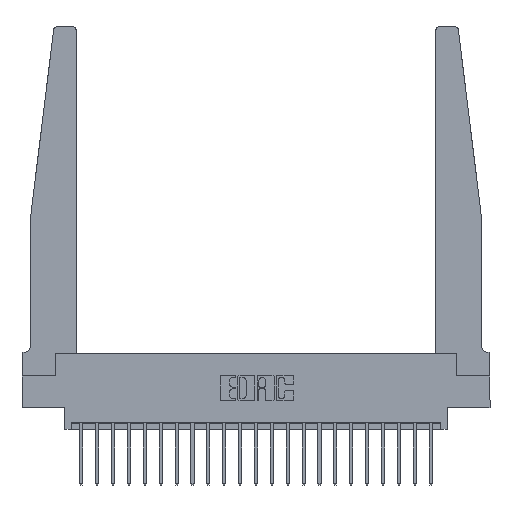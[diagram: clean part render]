
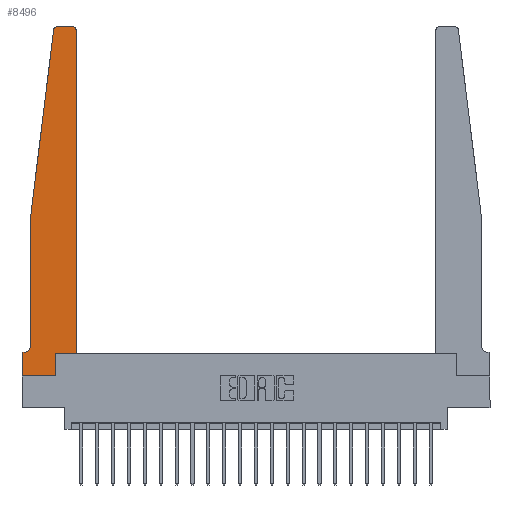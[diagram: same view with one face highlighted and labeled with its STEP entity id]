
A CAD part, top view. The second image highlights one B-rep face of the part: STEP entity #8496.
In plain terms, the highlighted planar face has unit normal (0, 0, 1).
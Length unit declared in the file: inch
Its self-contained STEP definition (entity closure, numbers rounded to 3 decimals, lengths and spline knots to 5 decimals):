
#109 = EDGE_LOOP ( 'NONE', ( #13309, #15903, #14687, #2676, #15433, #5924, #4441, #11190, #1100, #531, #7987, #18024 ) ) ;
#251 = CARTESIAN_POINT ( 'NONE',  ( 0.425, 2.72, 0.37 ) ) ;
#488 = EDGE_CURVE ( 'NONE', #21407, #11860, #6387, .T. ) ;
#531 = ORIENTED_EDGE ( 'NONE', *, *, #16095, .T. ) ;
#1100 = ORIENTED_EDGE ( 'NONE', *, *, #2071, .T. ) ;
#1264 = DIRECTION ( 'NONE',  ( -1., 0., 0. ) ) ;
#1304 = VECTOR ( 'NONE', #15452, 39.37008 ) ;
#2071 = EDGE_CURVE ( 'NONE', #9517, #12862, #4675, .T. ) ;
#2253 = CARTESIAN_POINT ( 'NONE',  ( 0., 0., 0.37 ) ) ;
#2350 = CIRCLE ( 'NONE', #16091, 0.05 ) ;
#2676 = ORIENTED_EDGE ( 'NONE', *, *, #9889, .T. ) ;
#2680 = VERTEX_POINT ( 'NONE', #2723 ) ;
#2683 = DIRECTION ( 'NONE',  ( 1., 0., 0. ) ) ;
#2723 = CARTESIAN_POINT ( 'NONE',  ( 0., 0.1875, 0.37 ) ) ;
#3309 = DIRECTION ( 'NONE',  ( 0., 0., 1. ) ) ;
#3748 = EDGE_CURVE ( 'NONE', #21565, #18708, #15026, .T. ) ;
#3820 = LINE ( 'NONE', #15959, #9066 ) ;
#4441 = ORIENTED_EDGE ( 'NONE', *, *, #20902, .T. ) ;
#4668 = CARTESIAN_POINT ( 'NONE',  ( 0.395, 2.72, 0.37 ) ) ;
#4675 = LINE ( 'NONE', #7971, #13459 ) ;
#4796 = CARTESIAN_POINT ( 'NONE',  ( 0.065, 1.25, 0.37 ) ) ;
#5577 = CARTESIAN_POINT ( 'NONE',  ( 0., 0., 0.37 ) ) ;
#5736 = CARTESIAN_POINT ( 'NONE',  ( 0.2605, 0.18, 0.37 ) ) ;
#5771 = CARTESIAN_POINT ( 'NONE',  ( 0.2605, 0., 0.37 ) ) ;
#5870 = LINE ( 'NONE', #11417, #14626 ) ;
#5924 = ORIENTED_EDGE ( 'NONE', *, *, #21323, .T. ) ;
#6345 = CARTESIAN_POINT ( 'NONE',  ( 0., 0., 0.37 ) ) ;
#6387 = LINE ( 'NONE', #19167, #15132 ) ;
#6426 = DIRECTION ( 'NONE',  ( 1., 0., 0. ) ) ;
#6917 = EDGE_CURVE ( 'NONE', #17270, #9517, #17255, .T. ) ;
#6974 = EDGE_CURVE ( 'NONE', #11742, #21407, #16705, .T. ) ;
#7062 = LINE ( 'NONE', #20667, #20421 ) ;
#7329 = DIRECTION ( 'NONE',  ( 0., -1., 0. ) ) ;
#7659 = LINE ( 'NONE', #5577, #16386 ) ;
#7971 = CARTESIAN_POINT ( 'NONE',  ( 0.2605, 0.18, 0.37 ) ) ;
#7987 = ORIENTED_EDGE ( 'NONE', *, *, #19603, .T. ) ;
#8454 = CARTESIAN_POINT ( 'NONE',  ( 0.25, 2.75, 0.37 ) ) ;
#8496 = ADVANCED_FACE ( 'NONE', ( #18513 ), #13808, .T. ) ;
#8518 = CARTESIAN_POINT ( 'NONE',  ( 0., 0.1875, 0.37 ) ) ;
#9066 = VECTOR ( 'NONE', #21141, 39.37008 ) ;
#9517 = VERTEX_POINT ( 'NONE', #5771 ) ;
#9761 = DIRECTION ( 'NONE',  ( 0., 1., 0. ) ) ;
#9889 = EDGE_CURVE ( 'NONE', #11860, #9933, #7062, .T. ) ;
#9890 = DIRECTION ( 'NONE',  ( 1., 0., 0. ) ) ;
#9933 = VERTEX_POINT ( 'NONE', #20735 ) ;
#10051 = CARTESIAN_POINT ( 'NONE',  ( 0.27653, 2.72, 0.37 ) ) ;
#10329 = DIRECTION ( 'NONE',  ( 0., -1., 0. ) ) ;
#11150 = VERTEX_POINT ( 'NONE', #20262 ) ;
#11190 = ORIENTED_EDGE ( 'NONE', *, *, #6917, .T. ) ;
#11417 = CARTESIAN_POINT ( 'NONE',  ( 0.425, 0.18, 0.37 ) ) ;
#11742 = VERTEX_POINT ( 'NONE', #13229 ) ;
#11788 = DIRECTION ( 'NONE',  ( 0., 0., -1. ) ) ;
#11811 = DIRECTION ( 'NONE',  ( 1., 0., 0. ) ) ;
#11853 = EDGE_CURVE ( 'NONE', #9933, #12474, #2350, .T. ) ;
#11860 = VERTEX_POINT ( 'NONE', #4796 ) ;
#11968 = CARTESIAN_POINT ( 'NONE',  ( 0.065, 0.1875, 0.37 ) ) ;
#12474 = VERTEX_POINT ( 'NONE', #22196 ) ;
#12680 = VECTOR ( 'NONE', #9890, 39.37008 ) ;
#12862 = VERTEX_POINT ( 'NONE', #5736 ) ;
#12879 = LINE ( 'NONE', #11968, #21466 ) ;
#13229 = CARTESIAN_POINT ( 'NONE',  ( 0.27653, 2.75, 0.37 ) ) ;
#13309 = ORIENTED_EDGE ( 'NONE', *, *, #22333, .T. ) ;
#13459 = VECTOR ( 'NONE', #9761, 39.37008 ) ;
#13808 = PLANE ( 'NONE',  #15047 ) ;
#13932 = CARTESIAN_POINT ( 'NONE',  ( 0.24675, 2.72367, 0.37 ) ) ;
#14626 = VECTOR ( 'NONE', #2683, 39.37008 ) ;
#14687 = ORIENTED_EDGE ( 'NONE', *, *, #488, .T. ) ;
#14810 = CARTESIAN_POINT ( 'NONE',  ( 0.395, 2.75, 0.37 ) ) ;
#15026 = CIRCLE ( 'NONE', #16412, 0.03 ) ;
#15047 = AXIS2_PLACEMENT_3D ( 'NONE', #8518, #3309, #15515 ) ;
#15132 = VECTOR ( 'NONE', #20918, 39.37008 ) ;
#15433 = ORIENTED_EDGE ( 'NONE', *, *, #11853, .T. ) ;
#15452 = DIRECTION ( 'NONE',  ( -1., 0., 0. ) ) ;
#15515 = DIRECTION ( 'NONE',  ( 1., 0., 0. ) ) ;
#15785 = LINE ( 'NONE', #8454, #1304 ) ;
#15903 = ORIENTED_EDGE ( 'NONE', *, *, #6974, .T. ) ;
#15959 = CARTESIAN_POINT ( 'NONE',  ( 0.425, 0.18, 0.37 ) ) ;
#16091 = AXIS2_PLACEMENT_3D ( 'NONE', #22061, #11788, #1264 ) ;
#16095 = EDGE_CURVE ( 'NONE', #12862, #11150, #5870, .T. ) ;
#16386 = VECTOR ( 'NONE', #7329, 39.37008 ) ;
#16412 = AXIS2_PLACEMENT_3D ( 'NONE', #4668, #16841, #6426 ) ;
#16705 = CIRCLE ( 'NONE', #21772, 0.03 ) ;
#16841 = DIRECTION ( 'NONE',  ( 0., 0., 1. ) ) ;
#17255 = LINE ( 'NONE', #6345, #12680 ) ;
#17270 = VERTEX_POINT ( 'NONE', #2253 ) ;
#18024 = ORIENTED_EDGE ( 'NONE', *, *, #3748, .T. ) ;
#18513 = FACE_OUTER_BOUND ( 'NONE', #109, .T. ) ;
#18708 = VERTEX_POINT ( 'NONE', #14810 ) ;
#19167 = CARTESIAN_POINT ( 'NONE',  ( 0.065, 1.25, 0.37 ) ) ;
#19603 = EDGE_CURVE ( 'NONE', #11150, #21565, #3820, .T. ) ;
#20262 = CARTESIAN_POINT ( 'NONE',  ( 0.425, 0.18, 0.37 ) ) ;
#20421 = VECTOR ( 'NONE', #10329, 39.37008 ) ;
#20667 = CARTESIAN_POINT ( 'NONE',  ( 0.065, 1.25, 0.37 ) ) ;
#20735 = CARTESIAN_POINT ( 'NONE',  ( 0.065, 0.2375, 0.37 ) ) ;
#20902 = EDGE_CURVE ( 'NONE', #2680, #17270, #7659, .T. ) ;
#20918 = DIRECTION ( 'NONE',  ( -0.122, -0.992, 0. ) ) ;
#21141 = DIRECTION ( 'NONE',  ( 0., 1., 0. ) ) ;
#21323 = EDGE_CURVE ( 'NONE', #12474, #2680, #12879, .T. ) ;
#21407 = VERTEX_POINT ( 'NONE', #13932 ) ;
#21466 = VECTOR ( 'NONE', #22238, 39.37008 ) ;
#21565 = VERTEX_POINT ( 'NONE', #251 ) ;
#21772 = AXIS2_PLACEMENT_3D ( 'NONE', #10051, #22085, #11811 ) ;
#22061 = CARTESIAN_POINT ( 'NONE',  ( 0.015, 0.2375, 0.37 ) ) ;
#22085 = DIRECTION ( 'NONE',  ( 0., 0., 1. ) ) ;
#22196 = CARTESIAN_POINT ( 'NONE',  ( 0.015, 0.1875, 0.37 ) ) ;
#22238 = DIRECTION ( 'NONE',  ( -1., 0., 0. ) ) ;
#22333 = EDGE_CURVE ( 'NONE', #18708, #11742, #15785, .T. ) ;
